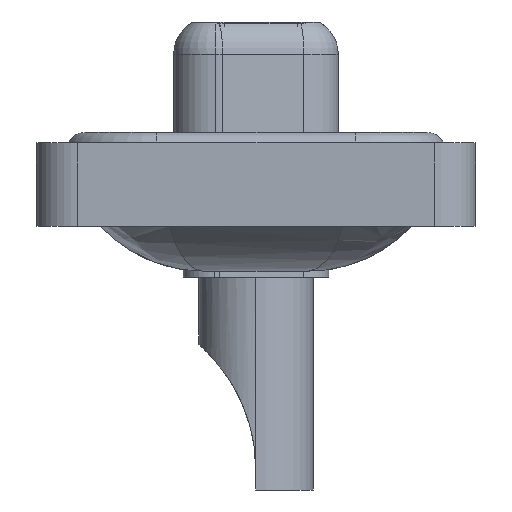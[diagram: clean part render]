
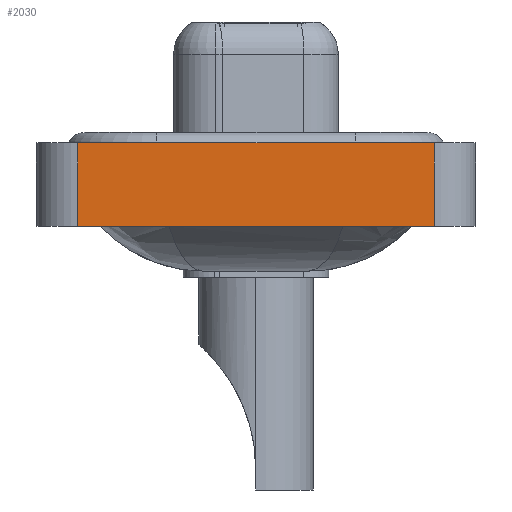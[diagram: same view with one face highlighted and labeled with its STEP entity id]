
A CAD part, left-side view. The second image highlights one B-rep face of the part: STEP entity #2030.
In plain terms, the highlighted planar face has unit normal (-1, 0, 0).
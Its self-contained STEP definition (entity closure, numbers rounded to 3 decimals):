
#564 = EDGE_CURVE ( 'NONE', #14527, #15173, #2222, .T. ) ;
#734 = DIRECTION ( 'NONE',  ( 0., -1., 0. ) ) ;
#886 = CARTESIAN_POINT ( 'NONE',  ( -7.35, -8.55, -3.6 ) ) ;
#1096 = VERTEX_POINT ( 'NONE', #6505 ) ;
#1485 = CARTESIAN_POINT ( 'NONE',  ( -7.35, 8.55, 0.4 ) ) ;
#1638 = LINE ( 'NONE', #13242, #6180 ) ;
#2030 = ADVANCED_FACE ( 'NONE', ( #11588 ), #15319, .T. ) ;
#2222 = LINE ( 'NONE', #7326, #10148 ) ;
#2396 = ORIENTED_EDGE ( 'NONE', *, *, #7435, .T. ) ;
#3473 = EDGE_CURVE ( 'NONE', #14527, #1096, #1638, .T. ) ;
#4686 = CARTESIAN_POINT ( 'NONE',  ( -7.35, -8.55, 0.4 ) ) ;
#5958 = DIRECTION ( 'NONE',  ( 0., -1., 0. ) ) ;
#6180 = VECTOR ( 'NONE', #734, 1000. ) ;
#6505 = CARTESIAN_POINT ( 'NONE',  ( -7.35, -8.55, -3.6 ) ) ;
#7034 = ORIENTED_EDGE ( 'NONE', *, *, #14747, .F. ) ;
#7326 = CARTESIAN_POINT ( 'NONE',  ( -7.35, 8.55, -3.6 ) ) ;
#7435 = EDGE_CURVE ( 'NONE', #1096, #15474, #10158, .T. ) ;
#7525 = VECTOR ( 'NONE', #8509, 1000. ) ;
#8509 = DIRECTION ( 'NONE',  ( 0., 0., 1. ) ) ;
#8559 = LINE ( 'NONE', #4686, #9941 ) ;
#9941 = VECTOR ( 'NONE', #5958, 1000. ) ;
#10148 = VECTOR ( 'NONE', #12409, 1000. ) ;
#10158 = LINE ( 'NONE', #886, #7525 ) ;
#10332 = DIRECTION ( 'NONE',  ( -1., 0., 0. ) ) ;
#10405 = CARTESIAN_POINT ( 'NONE',  ( -7.35, -8.55, -3.6 ) ) ;
#11588 = FACE_OUTER_BOUND ( 'NONE', #13670, .T. ) ;
#11887 = CARTESIAN_POINT ( 'NONE',  ( -7.35, -8.55, 0.4 ) ) ;
#11960 = CARTESIAN_POINT ( 'NONE',  ( -7.35, 8.55, -3.6 ) ) ;
#12409 = DIRECTION ( 'NONE',  ( 0., 0., 1. ) ) ;
#12584 = DIRECTION ( 'NONE',  ( 0., 0., 1. ) ) ;
#12962 = ORIENTED_EDGE ( 'NONE', *, *, #3473, .T. ) ;
#13242 = CARTESIAN_POINT ( 'NONE',  ( -7.35, -8.55, -3.6 ) ) ;
#13670 = EDGE_LOOP ( 'NONE', ( #2396, #7034, #16188, #12962 ) ) ;
#14527 = VERTEX_POINT ( 'NONE', #11960 ) ;
#14747 = EDGE_CURVE ( 'NONE', #15173, #15474, #8559, .T. ) ;
#15173 = VERTEX_POINT ( 'NONE', #1485 ) ;
#15319 = PLANE ( 'NONE',  #15990 ) ;
#15474 = VERTEX_POINT ( 'NONE', #11887 ) ;
#15990 = AXIS2_PLACEMENT_3D ( 'NONE', #10405, #10332, #12584 ) ;
#16188 = ORIENTED_EDGE ( 'NONE', *, *, #564, .F. ) ;
